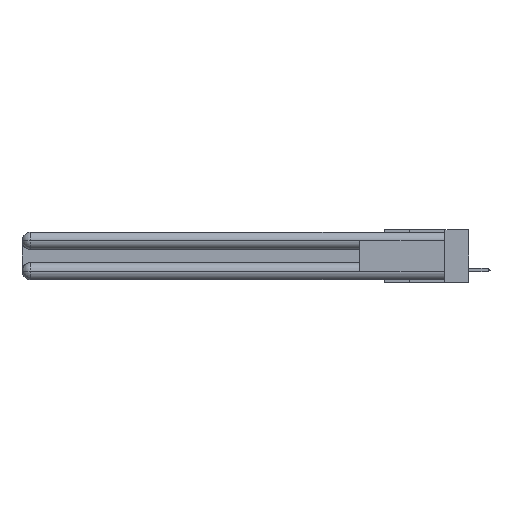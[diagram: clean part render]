
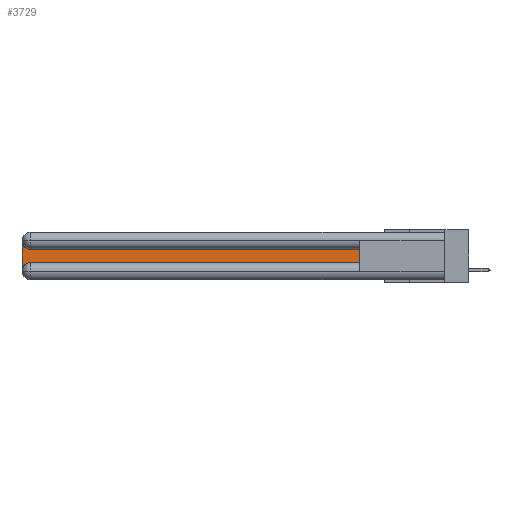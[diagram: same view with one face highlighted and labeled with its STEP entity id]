
A CAD part, left-side view. The second image highlights one B-rep face of the part: STEP entity #3729.
In plain terms, the highlighted planar face has unit normal (-1, 0, 0).
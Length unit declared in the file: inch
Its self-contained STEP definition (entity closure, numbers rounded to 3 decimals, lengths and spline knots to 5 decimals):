
#510 = DIRECTION ( 'NONE',  ( 0., 0., -1. ) ) ;
#512 = CARTESIAN_POINT ( 'NONE',  ( 0.075, 2.94, -0.0625 ) ) ;
#1116 = ORIENTED_EDGE ( 'NONE', *, *, #19942, .T. ) ;
#1490 = ORIENTED_EDGE ( 'NONE', *, *, #15669, .T. ) ;
#1538 = CARTESIAN_POINT ( 'NONE',  ( 0.075, 3., -0.0625 ) ) ;
#1595 = CARTESIAN_POINT ( 'NONE',  ( 0.075, 0.6, -0.1225 ) ) ;
#2328 = CIRCLE ( 'NONE', #10729, 0.06 ) ;
#2614 = FACE_OUTER_BOUND ( 'NONE', #27946, .T. ) ;
#2899 = EDGE_CURVE ( 'NONE', #9651, #15450, #24559, .T. ) ;
#2966 = DIRECTION ( 'NONE',  ( 1., 0., 0. ) ) ;
#3269 = CARTESIAN_POINT ( 'NONE',  ( 0.075, 2.94, -0.2775 ) ) ;
#3729 = ADVANCED_FACE ( 'NONE', ( #2614 ), #18247, .F. ) ;
#4088 = AXIS2_PLACEMENT_3D ( 'NONE', #20389, #4278, #4160 ) ;
#4160 = DIRECTION ( 'NONE',  ( 0., 0., -1. ) ) ;
#4278 = DIRECTION ( 'NONE',  ( 1., 0., 0. ) ) ;
#4852 = VECTOR ( 'NONE', #11362, 39.37008 ) ;
#5165 = DIRECTION ( 'NONE',  ( 0., 0., -1. ) ) ;
#5584 = LINE ( 'NONE', #22900, #4852 ) ;
#6358 = VECTOR ( 'NONE', #510, 39.37008 ) ;
#6870 = VERTEX_POINT ( 'NONE', #1538 ) ;
#8576 = VECTOR ( 'NONE', #12401, 39.37008 ) ;
#9508 = CARTESIAN_POINT ( 'NONE',  ( 0.075, 2.94, -0.1225 ) ) ;
#9609 = VERTEX_POINT ( 'NONE', #9508 ) ;
#9651 = VERTEX_POINT ( 'NONE', #21037 ) ;
#9834 = CARTESIAN_POINT ( 'NONE',  ( 0.075, 0.6, -0.1225 ) ) ;
#10299 = DIRECTION ( 'NONE',  ( 0., 0., -1. ) ) ;
#10729 = AXIS2_PLACEMENT_3D ( 'NONE', #512, #21572, #5165 ) ;
#11193 = EDGE_CURVE ( 'NONE', #15627, #9609, #23863, .T. ) ;
#11362 = DIRECTION ( 'NONE',  ( 0., -1., 0. ) ) ;
#12401 = DIRECTION ( 'NONE',  ( 0., 0., 1. ) ) ;
#12528 = VERTEX_POINT ( 'NONE', #13753 ) ;
#13753 = CARTESIAN_POINT ( 'NONE',  ( 0.075, 0.6, -0.2175 ) ) ;
#13938 = ORIENTED_EDGE ( 'NONE', *, *, #11193, .T. ) ;
#15450 = VERTEX_POINT ( 'NONE', #19970 ) ;
#15468 = VECTOR ( 'NONE', #17945, 39.37008 ) ;
#15627 = VERTEX_POINT ( 'NONE', #9834 ) ;
#15669 = EDGE_CURVE ( 'NONE', #9609, #6870, #2328, .T. ) ;
#17197 = CARTESIAN_POINT ( 'NONE',  ( 0.075, 0.6, -0.2175 ) ) ;
#17754 = AXIS2_PLACEMENT_3D ( 'NONE', #3269, #2966, #10299 ) ;
#17945 = DIRECTION ( 'NONE',  ( 0., 1., 0. ) ) ;
#18247 = PLANE ( 'NONE',  #4088 ) ;
#19244 = ORIENTED_EDGE ( 'NONE', *, *, #27299, .T. ) ;
#19942 = EDGE_CURVE ( 'NONE', #6870, #9651, #29393, .T. ) ;
#19970 = CARTESIAN_POINT ( 'NONE',  ( 0.075, 2.94, -0.2175 ) ) ;
#20389 = CARTESIAN_POINT ( 'NONE',  ( 0.075, 3., -0.1225 ) ) ;
#21037 = CARTESIAN_POINT ( 'NONE',  ( 0.075, 3., -0.2775 ) ) ;
#21324 = LINE ( 'NONE', #17197, #8576 ) ;
#21572 = DIRECTION ( 'NONE',  ( 1., 0., 0. ) ) ;
#21592 = EDGE_CURVE ( 'NONE', #15450, #12528, #5584, .T. ) ;
#22900 = CARTESIAN_POINT ( 'NONE',  ( 0.075, 0.6, -0.2175 ) ) ;
#23863 = LINE ( 'NONE', #1595, #15468 ) ;
#24559 = CIRCLE ( 'NONE', #17754, 0.06 ) ;
#24935 = ORIENTED_EDGE ( 'NONE', *, *, #2899, .T. ) ;
#27004 = ORIENTED_EDGE ( 'NONE', *, *, #21592, .T. ) ;
#27299 = EDGE_CURVE ( 'NONE', #12528, #15627, #21324, .T. ) ;
#27924 = CARTESIAN_POINT ( 'NONE',  ( 0.075, 3., -0.2175 ) ) ;
#27946 = EDGE_LOOP ( 'NONE', ( #13938, #1490, #1116, #24935, #27004, #19244 ) ) ;
#29393 = LINE ( 'NONE', #27924, #6358 ) ;
